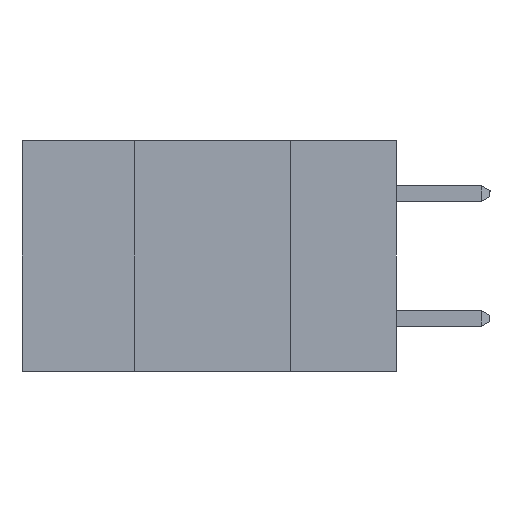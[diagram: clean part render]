
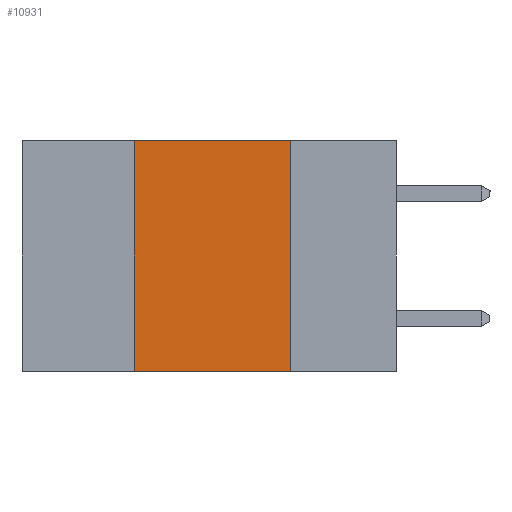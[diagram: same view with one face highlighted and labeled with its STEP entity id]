
A CAD part, left-side view. The second image highlights one B-rep face of the part: STEP entity #10931.
In plain terms, the highlighted planar face has unit normal (-1, 0, 0).
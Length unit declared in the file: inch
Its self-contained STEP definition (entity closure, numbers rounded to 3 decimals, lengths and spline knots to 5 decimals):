
#596 = EDGE_LOOP ( 'NONE', ( #9767, #4474, #9442, #12735 ) ) ;
#832 = VERTEX_POINT ( 'NONE', #8859 ) ;
#1593 = DIRECTION ( 'NONE',  ( 1., 0., 0. ) ) ;
#1623 = VERTEX_POINT ( 'NONE', #14631 ) ;
#1709 = CARTESIAN_POINT ( 'NONE',  ( 0., 0.6, 0. ) ) ;
#2268 = CARTESIAN_POINT ( 'NONE',  ( 0., 0.6, 0. ) ) ;
#3661 = CARTESIAN_POINT ( 'NONE',  ( 0., 0.42, -0.37 ) ) ;
#4153 = EDGE_CURVE ( 'NONE', #20631, #9709, #20205, .T. ) ;
#4474 = ORIENTED_EDGE ( 'NONE', *, *, #10098, .F. ) ;
#4479 = CARTESIAN_POINT ( 'NONE',  ( 0., 0.17, -0.37 ) ) ;
#4649 = DIRECTION ( 'NONE',  ( 0., -1., 0. ) ) ;
#5245 = FACE_OUTER_BOUND ( 'NONE', #596, .T. ) ;
#7099 = CARTESIAN_POINT ( 'NONE',  ( 0., 0.42, -0.37 ) ) ;
#7462 = CARTESIAN_POINT ( 'NONE',  ( 0., 0.42, 0. ) ) ;
#8859 = CARTESIAN_POINT ( 'NONE',  ( 0., 0.17, -0.37 ) ) ;
#8893 = DIRECTION ( 'NONE',  ( 0., 0., -1. ) ) ;
#9415 = DIRECTION ( 'NONE',  ( 0., 0., 1. ) ) ;
#9442 = ORIENTED_EDGE ( 'NONE', *, *, #4153, .F. ) ;
#9709 = VERTEX_POINT ( 'NONE', #7462 ) ;
#9767 = ORIENTED_EDGE ( 'NONE', *, *, #12809, .F. ) ;
#10001 = DIRECTION ( 'NONE',  ( 0., 0., -1. ) ) ;
#10098 = EDGE_CURVE ( 'NONE', #9709, #1623, #11215, .T. ) ;
#10809 = VECTOR ( 'NONE', #4649, 39.37008 ) ;
#10931 = ADVANCED_FACE ( 'NONE', ( #5245 ), #17693, .F. ) ;
#11215 = LINE ( 'NONE', #2268, #17422 ) ;
#12735 = ORIENTED_EDGE ( 'NONE', *, *, #15914, .T. ) ;
#12809 = EDGE_CURVE ( 'NONE', #1623, #832, #13406, .T. ) ;
#13406 = LINE ( 'NONE', #4479, #23156 ) ;
#14631 = CARTESIAN_POINT ( 'NONE',  ( 0., 0.17, 0. ) ) ;
#14725 = DIRECTION ( 'NONE',  ( 0., -1., 0. ) ) ;
#15914 = EDGE_CURVE ( 'NONE', #20631, #832, #17207, .T. ) ;
#17207 = LINE ( 'NONE', #22513, #10809 ) ;
#17422 = VECTOR ( 'NONE', #14725, 39.37008 ) ;
#17693 = PLANE ( 'NONE',  #21964 ) ;
#18359 = VECTOR ( 'NONE', #9415, 39.37008 ) ;
#20205 = LINE ( 'NONE', #3661, #18359 ) ;
#20631 = VERTEX_POINT ( 'NONE', #7099 ) ;
#21964 = AXIS2_PLACEMENT_3D ( 'NONE', #1709, #1593, #8893 ) ;
#22513 = CARTESIAN_POINT ( 'NONE',  ( 0., 0.6, -0.37 ) ) ;
#23156 = VECTOR ( 'NONE', #10001, 39.37008 ) ;
